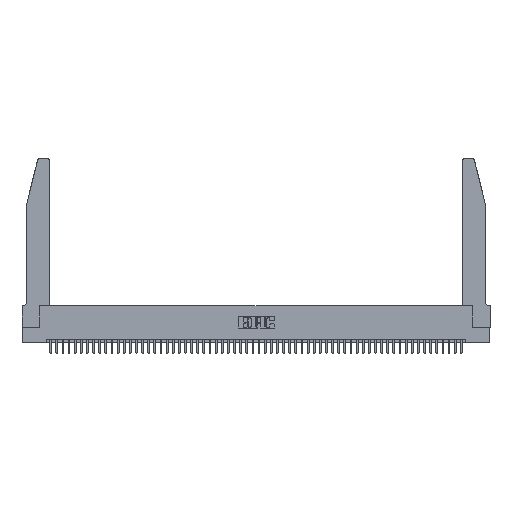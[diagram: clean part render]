
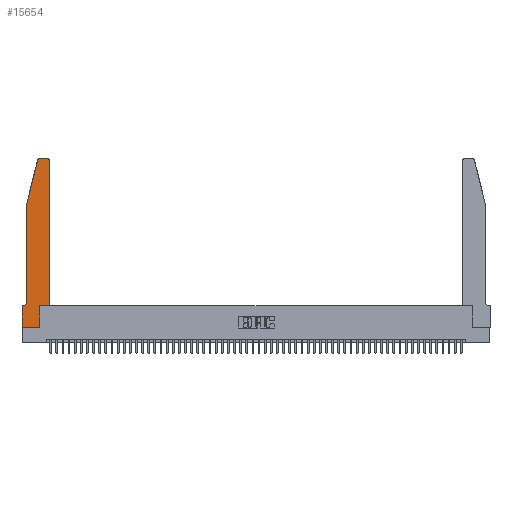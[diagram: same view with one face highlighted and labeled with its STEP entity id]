
A CAD part, top view. The second image highlights one B-rep face of the part: STEP entity #15654.
In plain terms, the highlighted planar face has unit normal (0, 0, 1).
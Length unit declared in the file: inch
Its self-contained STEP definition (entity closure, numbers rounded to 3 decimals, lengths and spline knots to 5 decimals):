
#165 = VECTOR ( 'NONE', #13881, 39.37008 ) ;
#1160 = CARTESIAN_POINT ( 'NONE',  ( 0.4505, 0.35, 0.37 ) ) ;
#1448 = CARTESIAN_POINT ( 'NONE',  ( 0.25487, 2.72718, 0.37 ) ) ;
#3578 = VERTEX_POINT ( 'NONE', #15085 ) ;
#4511 = VECTOR ( 'NONE', #21743, 39.37008 ) ;
#4798 = VERTEX_POINT ( 'NONE', #53381 ) ;
#5601 = EDGE_CURVE ( 'NONE', #52168, #13221, #15256, .T. ) ;
#5745 = DIRECTION ( 'NONE',  ( 0., 0., 1. ) ) ;
#6115 = CARTESIAN_POINT ( 'NONE',  ( 0., 0.35, 0.37 ) ) ;
#6135 = FACE_OUTER_BOUND ( 'NONE', #51707, .T. ) ;
#6396 = CARTESIAN_POINT ( 'NONE',  ( 0.4505, 0.35, 0.37 ) ) ;
#7976 = AXIS2_PLACEMENT_3D ( 'NONE', #6115, #18874, #48437 ) ;
#8145 = ORIENTED_EDGE ( 'NONE', *, *, #14163, .T. ) ;
#8538 = CARTESIAN_POINT ( 'NONE',  ( 0.2605, 2.75, 0.37 ) ) ;
#8662 = CARTESIAN_POINT ( 'NONE',  ( 0.284, 2.75, 0.37 ) ) ;
#8844 = VERTEX_POINT ( 'NONE', #1160 ) ;
#9619 = CARTESIAN_POINT ( 'NONE',  ( 0.0755, 2., 0.37 ) ) ;
#10032 = EDGE_CURVE ( 'NONE', #14387, #37864, #35942, .T. ) ;
#10221 = VECTOR ( 'NONE', #19166, 39.37008 ) ;
#11106 = CARTESIAN_POINT ( 'NONE',  ( 0.4505, 0.35, 0.37 ) ) ;
#11550 = LINE ( 'NONE', #6396, #10221 ) ;
#11572 = EDGE_CURVE ( 'NONE', #13221, #8844, #39083, .T. ) ;
#11694 = CARTESIAN_POINT ( 'NONE',  ( 0.0055, 0.35, 0.37 ) ) ;
#13043 = CARTESIAN_POINT ( 'NONE',  ( 0.2865, 0.35, 0.37 ) ) ;
#13221 = VERTEX_POINT ( 'NONE', #26097 ) ;
#13881 = DIRECTION ( 'NONE',  ( -0.239, -0.971, 0. ) ) ;
#14163 = EDGE_CURVE ( 'NONE', #44496, #52168, #21569, .T. ) ;
#14387 = VERTEX_POINT ( 'NONE', #18179 ) ;
#15085 = CARTESIAN_POINT ( 'NONE',  ( 0.4505, 2.72, 0.37 ) ) ;
#15256 = LINE ( 'NONE', #13043, #36453 ) ;
#15259 = VERTEX_POINT ( 'NONE', #11694 ) ;
#15539 = EDGE_CURVE ( 'NONE', #47987, #14387, #45231, .T. ) ;
#15654 = ADVANCED_FACE ( 'NONE', ( #6135 ), #44239, .T. ) ;
#16587 = EDGE_CURVE ( 'NONE', #4798, #44496, #36566, .T. ) ;
#17056 = CARTESIAN_POINT ( 'NONE',  ( 0.4205, 2.72, 0.37 ) ) ;
#17294 = DIRECTION ( 'NONE',  ( 0., 1., 0. ) ) ;
#17379 = CARTESIAN_POINT ( 'NONE',  ( 0.0755, 2., 0.37 ) ) ;
#18179 = CARTESIAN_POINT ( 'NONE',  ( 0.0755, 2., 0.37 ) ) ;
#18367 = ORIENTED_EDGE ( 'NONE', *, *, #32397, .T. ) ;
#18444 = CARTESIAN_POINT ( 'NONE',  ( 0.4205, 2.75, 0.37 ) ) ;
#18874 = DIRECTION ( 'NONE',  ( 0., 0., 1. ) ) ;
#19166 = DIRECTION ( 'NONE',  ( 0., 1., 0. ) ) ;
#20066 = CIRCLE ( 'NONE', #25855, 0.07 ) ;
#20116 = CARTESIAN_POINT ( 'NONE',  ( 0., 0., 0.37 ) ) ;
#21030 = CARTESIAN_POINT ( 'NONE',  ( 0.0055, 0.42, 0.37 ) ) ;
#21365 = DIRECTION ( 'NONE',  ( 1., 0., 0. ) ) ;
#21569 = LINE ( 'NONE', #36326, #32781 ) ;
#21668 = DIRECTION ( 'NONE',  ( 0., -1., 0. ) ) ;
#21743 = DIRECTION ( 'NONE',  ( -1., 0., 0. ) ) ;
#21903 = AXIS2_PLACEMENT_3D ( 'NONE', #31102, #5745, #35366 ) ;
#22365 = VECTOR ( 'NONE', #42422, 39.37008 ) ;
#23490 = EDGE_CURVE ( 'NONE', #3578, #49316, #39192, .T. ) ;
#23758 = DIRECTION ( 'NONE',  ( 1., 0., 0. ) ) ;
#24089 = DIRECTION ( 'NONE',  ( 1., 0., 0. ) ) ;
#25174 = ORIENTED_EDGE ( 'NONE', *, *, #23490, .T. ) ;
#25262 = DIRECTION ( 'NONE',  ( -1., 0., 0. ) ) ;
#25334 = VECTOR ( 'NONE', #28624, 39.37008 ) ;
#25855 = AXIS2_PLACEMENT_3D ( 'NONE', #21030, #50552, #25262 ) ;
#26044 = VECTOR ( 'NONE', #21668, 39.37008 ) ;
#26097 = CARTESIAN_POINT ( 'NONE',  ( 0.2865, 0.35, 0.37 ) ) ;
#26513 = VECTOR ( 'NONE', #24089, 39.37008 ) ;
#26576 = CARTESIAN_POINT ( 'NONE',  ( 0.0755, 0.42, 0.37 ) ) ;
#26909 = ORIENTED_EDGE ( 'NONE', *, *, #33544, .T. ) ;
#27333 = ORIENTED_EDGE ( 'NONE', *, *, #11572, .T. ) ;
#28624 = DIRECTION ( 'NONE',  ( 0., -1., 0. ) ) ;
#31102 = CARTESIAN_POINT ( 'NONE',  ( 0.284, 2.72, 0.37 ) ) ;
#32397 = EDGE_CURVE ( 'NONE', #8844, #3578, #11550, .T. ) ;
#32781 = VECTOR ( 'NONE', #23758, 39.37008 ) ;
#33544 = EDGE_CURVE ( 'NONE', #49316, #36160, #47505, .T. ) ;
#33660 = CARTESIAN_POINT ( 'NONE',  ( 0., 0., 0.37 ) ) ;
#35366 = DIRECTION ( 'NONE',  ( 1., 0., 0. ) ) ;
#35942 = LINE ( 'NONE', #17379, #26044 ) ;
#36160 = VERTEX_POINT ( 'NONE', #8662 ) ;
#36326 = CARTESIAN_POINT ( 'NONE',  ( 0., 0., 0.37 ) ) ;
#36453 = VECTOR ( 'NONE', #17294, 39.37008 ) ;
#36566 = LINE ( 'NONE', #20116, #25334 ) ;
#37864 = VERTEX_POINT ( 'NONE', #26576 ) ;
#38526 = ORIENTED_EDGE ( 'NONE', *, *, #15539, .T. ) ;
#39083 = LINE ( 'NONE', #11106, #26513 ) ;
#39192 = CIRCLE ( 'NONE', #39424, 0.03 ) ;
#39424 = AXIS2_PLACEMENT_3D ( 'NONE', #17056, #46678, #21365 ) ;
#40330 = ORIENTED_EDGE ( 'NONE', *, *, #53074, .T. ) ;
#40570 = ORIENTED_EDGE ( 'NONE', *, *, #47340, .T. ) ;
#40767 = ORIENTED_EDGE ( 'NONE', *, *, #50531, .T. ) ;
#41630 = ORIENTED_EDGE ( 'NONE', *, *, #10032, .T. ) ;
#42422 = DIRECTION ( 'NONE',  ( -1., 0., 0. ) ) ;
#44239 = PLANE ( 'NONE',  #7976 ) ;
#44496 = VERTEX_POINT ( 'NONE', #33660 ) ;
#45231 = LINE ( 'NONE', #9619, #165 ) ;
#46678 = DIRECTION ( 'NONE',  ( 0., 0., 1. ) ) ;
#46883 = LINE ( 'NONE', #47058, #4511 ) ;
#47030 = ORIENTED_EDGE ( 'NONE', *, *, #16587, .T. ) ;
#47058 = CARTESIAN_POINT ( 'NONE',  ( 0.0755, 0.35, 0.37 ) ) ;
#47340 = EDGE_CURVE ( 'NONE', #15259, #4798, #46883, .T. ) ;
#47505 = LINE ( 'NONE', #8538, #22365 ) ;
#47987 = VERTEX_POINT ( 'NONE', #1448 ) ;
#48437 = DIRECTION ( 'NONE',  ( 1., 0., 0. ) ) ;
#48783 = CARTESIAN_POINT ( 'NONE',  ( 0.2865, 0., 0.37 ) ) ;
#49316 = VERTEX_POINT ( 'NONE', #18444 ) ;
#50454 = CIRCLE ( 'NONE', #21903, 0.03 ) ;
#50531 = EDGE_CURVE ( 'NONE', #36160, #47987, #50454, .T. ) ;
#50552 = DIRECTION ( 'NONE',  ( 0., 0., -1. ) ) ;
#51707 = EDGE_LOOP ( 'NONE', ( #26909, #40767, #38526, #41630, #40330, #40570, #47030, #8145, #54704, #27333, #18367, #25174 ) ) ;
#52168 = VERTEX_POINT ( 'NONE', #48783 ) ;
#53074 = EDGE_CURVE ( 'NONE', #37864, #15259, #20066, .T. ) ;
#53381 = CARTESIAN_POINT ( 'NONE',  ( 0., 0.35, 0.37 ) ) ;
#54704 = ORIENTED_EDGE ( 'NONE', *, *, #5601, .T. ) ;
